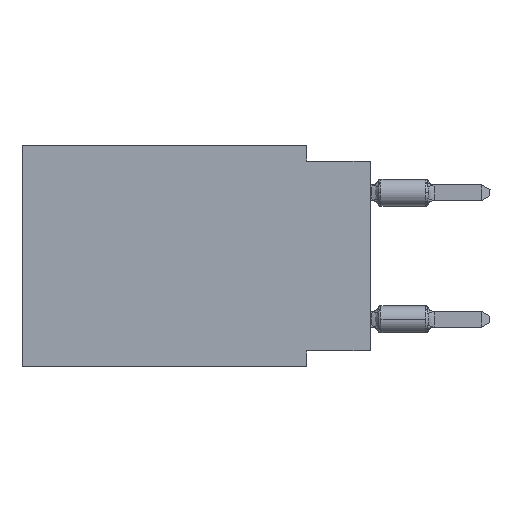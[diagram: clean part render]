
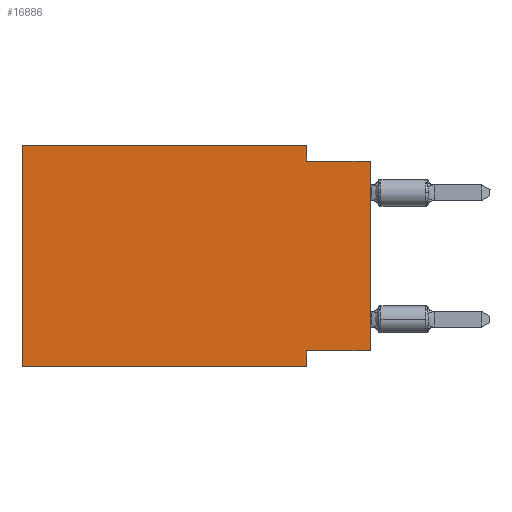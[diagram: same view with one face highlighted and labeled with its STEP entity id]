
A CAD part, left-side view. The second image highlights one B-rep face of the part: STEP entity #16886.
In plain terms, the highlighted planar face has unit normal (-1, 0, 0).
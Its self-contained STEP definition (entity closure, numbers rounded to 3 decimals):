
#449 = VERTEX_POINT ( 'NONE', #3955 ) ;
#682 = AXIS2_PLACEMENT_3D ( 'NONE', #7526, #9227, #26375 ) ;
#783 = EDGE_LOOP ( 'NONE', ( #15276, #19308, #11472, #4568, #8026, #3928, #18021, #17245 ) ) ;
#1258 = EDGE_CURVE ( 'NONE', #449, #3301, #1895, .T. ) ;
#1436 = VECTOR ( 'NONE', #15592, 1000. ) ;
#1565 = CARTESIAN_POINT ( 'NONE',  ( 0., 2.54, -0.635 ) ) ;
#1895 = LINE ( 'NONE', #10476, #6665 ) ;
#2593 = CARTESIAN_POINT ( 'NONE',  ( 0., 2.54, -8.89 ) ) ;
#2738 = PLANE ( 'NONE',  #682 ) ;
#2985 = VECTOR ( 'NONE', #20784, 1000. ) ;
#3301 = VERTEX_POINT ( 'NONE', #24942 ) ;
#3928 = ORIENTED_EDGE ( 'NONE', *, *, #22553, .T. ) ;
#3955 = CARTESIAN_POINT ( 'NONE',  ( 0., 13.97, -8.89 ) ) ;
#4425 = VERTEX_POINT ( 'NONE', #4580 ) ;
#4568 = ORIENTED_EDGE ( 'NONE', *, *, #6705, .F. ) ;
#4580 = CARTESIAN_POINT ( 'NONE',  ( 0., 0., -0.635 ) ) ;
#5907 = VECTOR ( 'NONE', #8437, 1000. ) ;
#6512 = DIRECTION ( 'NONE',  ( 0., 1., 0. ) ) ;
#6576 = CARTESIAN_POINT ( 'NONE',  ( 0., 2.54, -8.255 ) ) ;
#6665 = VECTOR ( 'NONE', #27772, 1000. ) ;
#6705 = EDGE_CURVE ( 'NONE', #3301, #27589, #17062, .T. ) ;
#7453 = VECTOR ( 'NONE', #23532, 1000. ) ;
#7526 = CARTESIAN_POINT ( 'NONE',  ( 0., 13.97, 0. ) ) ;
#8026 = ORIENTED_EDGE ( 'NONE', *, *, #1258, .F. ) ;
#8303 = LINE ( 'NONE', #21246, #5907 ) ;
#8437 = DIRECTION ( 'NONE',  ( 0., -1., 0. ) ) ;
#8559 = CARTESIAN_POINT ( 'NONE',  ( 0., 2.54, -8.89 ) ) ;
#8606 = VECTOR ( 'NONE', #6512, 1000. ) ;
#8768 = DIRECTION ( 'NONE',  ( 0., -1., 0. ) ) ;
#8827 = EDGE_CURVE ( 'NONE', #27589, #23718, #24443, .T. ) ;
#9227 = DIRECTION ( 'NONE',  ( 1., 0., 0. ) ) ;
#10421 = VECTOR ( 'NONE', #8768, 1000. ) ;
#10476 = CARTESIAN_POINT ( 'NONE',  ( 0., 13.97, 0. ) ) ;
#10792 = VERTEX_POINT ( 'NONE', #24051 ) ;
#11008 = LINE ( 'NONE', #19579, #8606 ) ;
#11234 = CARTESIAN_POINT ( 'NONE',  ( 0., 2.54, 0. ) ) ;
#11472 = ORIENTED_EDGE ( 'NONE', *, *, #8827, .F. ) ;
#11983 = EDGE_CURVE ( 'NONE', #23718, #4425, #15102, .T. ) ;
#12443 = EDGE_CURVE ( 'NONE', #20464, #21902, #13199, .T. ) ;
#12745 = EDGE_CURVE ( 'NONE', #10792, #4425, #18539, .T. ) ;
#13199 = LINE ( 'NONE', #8559, #20483 ) ;
#15102 = LINE ( 'NONE', #23671, #7453 ) ;
#15276 = ORIENTED_EDGE ( 'NONE', *, *, #12745, .T. ) ;
#15592 = DIRECTION ( 'NONE',  ( 0., 0., -1. ) ) ;
#16886 = ADVANCED_FACE ( 'NONE', ( #22012 ), #2738, .F. ) ;
#17062 = LINE ( 'NONE', #27469, #10421 ) ;
#17245 = ORIENTED_EDGE ( 'NONE', *, *, #23418, .F. ) ;
#18021 = ORIENTED_EDGE ( 'NONE', *, *, #12443, .F. ) ;
#18250 = DIRECTION ( 'NONE',  ( 0., 0., -1. ) ) ;
#18539 = LINE ( 'NONE', #25139, #2985 ) ;
#19308 = ORIENTED_EDGE ( 'NONE', *, *, #11983, .F. ) ;
#19579 = CARTESIAN_POINT ( 'NONE',  ( 0., 0., -8.255 ) ) ;
#20464 = VERTEX_POINT ( 'NONE', #6576 ) ;
#20483 = VECTOR ( 'NONE', #18250, 1000. ) ;
#20784 = DIRECTION ( 'NONE',  ( 0., 0., 1. ) ) ;
#21246 = CARTESIAN_POINT ( 'NONE',  ( 0., 13.97, -8.89 ) ) ;
#21902 = VERTEX_POINT ( 'NONE', #2593 ) ;
#22012 = FACE_OUTER_BOUND ( 'NONE', #783, .T. ) ;
#22553 = EDGE_CURVE ( 'NONE', #449, #21902, #8303, .T. ) ;
#23418 = EDGE_CURVE ( 'NONE', #10792, #20464, #11008, .T. ) ;
#23532 = DIRECTION ( 'NONE',  ( 0., -1., 0. ) ) ;
#23671 = CARTESIAN_POINT ( 'NONE',  ( 0., 0., -0.635 ) ) ;
#23718 = VERTEX_POINT ( 'NONE', #1565 ) ;
#23827 = CARTESIAN_POINT ( 'NONE',  ( 0., 2.54, 0. ) ) ;
#24051 = CARTESIAN_POINT ( 'NONE',  ( 0., 0., -8.255 ) ) ;
#24443 = LINE ( 'NONE', #11234, #1436 ) ;
#24942 = CARTESIAN_POINT ( 'NONE',  ( 0., 13.97, 0. ) ) ;
#25139 = CARTESIAN_POINT ( 'NONE',  ( 0., 0., 0. ) ) ;
#26375 = DIRECTION ( 'NONE',  ( 0., 0., -1. ) ) ;
#27469 = CARTESIAN_POINT ( 'NONE',  ( 0., 13.97, 0. ) ) ;
#27589 = VERTEX_POINT ( 'NONE', #23827 ) ;
#27772 = DIRECTION ( 'NONE',  ( 0., 0., 1. ) ) ;
